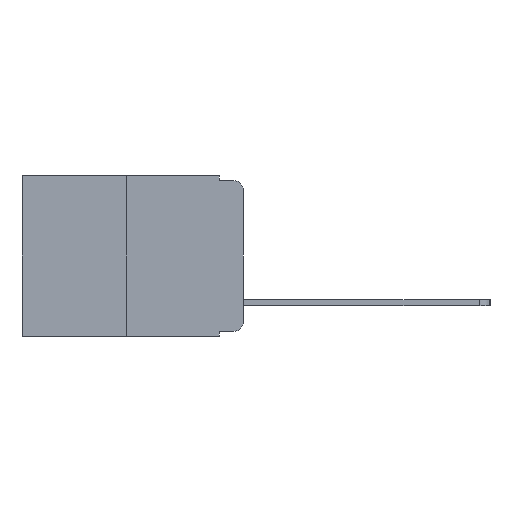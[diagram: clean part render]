
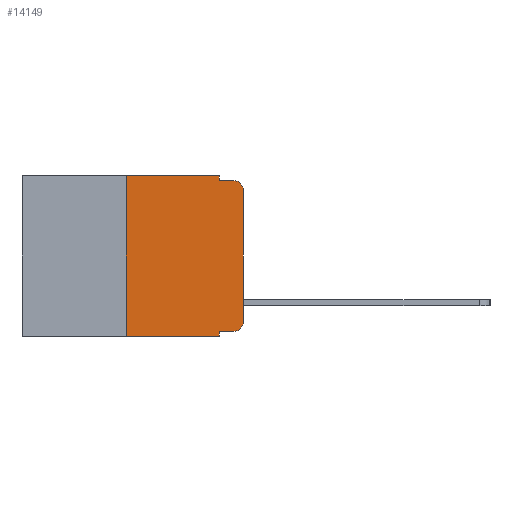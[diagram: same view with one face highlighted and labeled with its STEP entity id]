
A CAD part, left-side view. The second image highlights one B-rep face of the part: STEP entity #14149.
In plain terms, the highlighted planar face has unit normal (-1, 0, 0).
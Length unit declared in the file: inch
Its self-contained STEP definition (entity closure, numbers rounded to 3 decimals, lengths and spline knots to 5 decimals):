
#68 = CARTESIAN_POINT ( 'NONE',  ( 0., 0.473, -0.343 ) ) ;
#138 = DIRECTION ( 'NONE',  ( -1., 0., 0. ) ) ;
#363 = VECTOR ( 'NONE', #20311, 39.37008 ) ;
#501 = EDGE_CURVE ( 'NONE', #15374, #21090, #3777, .T. ) ;
#594 = CARTESIAN_POINT ( 'NONE',  ( 0., 0.02, -0.03 ) ) ;
#913 = ORIENTED_EDGE ( 'NONE', *, *, #1775, .T. ) ;
#965 = DIRECTION ( 'NONE',  ( 0., 0., -1. ) ) ;
#1468 = CIRCLE ( 'NONE', #21874, 0.02 ) ;
#1775 = EDGE_CURVE ( 'NONE', #3227, #13950, #23199, .T. ) ;
#1948 = VECTOR ( 'NONE', #9730, 39.37008 ) ;
#2402 = ORIENTED_EDGE ( 'NONE', *, *, #15412, .T. ) ;
#2527 = DIRECTION ( 'NONE',  ( 0., 0., -1. ) ) ;
#2558 = CARTESIAN_POINT ( 'NONE',  ( 0., 0.02, -0.333 ) ) ;
#3049 = EDGE_CURVE ( 'NONE', #13950, #14395, #9987, .T. ) ;
#3227 = VERTEX_POINT ( 'NONE', #12447 ) ;
#3551 = ORIENTED_EDGE ( 'NONE', *, *, #21712, .F. ) ;
#3776 = CARTESIAN_POINT ( 'NONE',  ( 0., 0.051, 0. ) ) ;
#3777 = LINE ( 'NONE', #68, #12321 ) ;
#3799 = LINE ( 'NONE', #8191, #17587 ) ;
#4627 = VERTEX_POINT ( 'NONE', #3776 ) ;
#5317 = DIRECTION ( 'NONE',  ( 0., 0., 1. ) ) ;
#5547 = EDGE_CURVE ( 'NONE', #3227, #21090, #6926, .T. ) ;
#5904 = CARTESIAN_POINT ( 'NONE',  ( 0., 0.051, -0.01 ) ) ;
#5955 = LINE ( 'NONE', #9815, #363 ) ;
#6106 = CARTESIAN_POINT ( 'NONE',  ( 0., 0.25, -0.343 ) ) ;
#6197 = ORIENTED_EDGE ( 'NONE', *, *, #18888, .T. ) ;
#6452 = CARTESIAN_POINT ( 'NONE',  ( 0., 0.051, -0.343 ) ) ;
#6875 = CARTESIAN_POINT ( 'NONE',  ( 0., 0.051, -0.01 ) ) ;
#6926 = LINE ( 'NONE', #7540, #1948 ) ;
#7183 = CARTESIAN_POINT ( 'NONE',  ( 0., 0., 0. ) ) ;
#7217 = VERTEX_POINT ( 'NONE', #16997 ) ;
#7333 = ORIENTED_EDGE ( 'NONE', *, *, #20123, .F. ) ;
#7540 = CARTESIAN_POINT ( 'NONE',  ( 0., 0.051, 0. ) ) ;
#7579 = VECTOR ( 'NONE', #11420, 39.37008 ) ;
#8191 = CARTESIAN_POINT ( 'NONE',  ( 0., 0.051, 0. ) ) ;
#8509 = ORIENTED_EDGE ( 'NONE', *, *, #13890, .F. ) ;
#8701 = DIRECTION ( 'NONE',  ( 0., -1., 0. ) ) ;
#9199 = VERTEX_POINT ( 'NONE', #5904 ) ;
#9230 = EDGE_CURVE ( 'NONE', #15374, #14036, #17061, .T. ) ;
#9583 = CARTESIAN_POINT ( 'NONE',  ( 0., 0.25, 0. ) ) ;
#9623 = ORIENTED_EDGE ( 'NONE', *, *, #5547, .F. ) ;
#9730 = DIRECTION ( 'NONE',  ( 0., 0., -1. ) ) ;
#9788 = VECTOR ( 'NONE', #13417, 39.37008 ) ;
#9815 = CARTESIAN_POINT ( 'NONE',  ( 0., 0.473, 0. ) ) ;
#9987 = CIRCLE ( 'NONE', #18444, 0.02 ) ;
#10115 = CARTESIAN_POINT ( 'NONE',  ( 0., 0.25, 0. ) ) ;
#10413 = DIRECTION ( 'NONE',  ( 1., 0., 0. ) ) ;
#10709 = ORIENTED_EDGE ( 'NONE', *, *, #3049, .T. ) ;
#11010 = LINE ( 'NONE', #6875, #15202 ) ;
#11275 = LINE ( 'NONE', #7183, #20554 ) ;
#11420 = DIRECTION ( 'NONE',  ( 0., 0., 1. ) ) ;
#12321 = VECTOR ( 'NONE', #15116, 39.37008 ) ;
#12447 = CARTESIAN_POINT ( 'NONE',  ( 0., 0.051, -0.333 ) ) ;
#13417 = DIRECTION ( 'NONE',  ( 0., -1., 0. ) ) ;
#13430 = DIRECTION ( 'NONE',  ( -1., 0., 0. ) ) ;
#13665 = CARTESIAN_POINT ( 'NONE',  ( 0., 0.051, -0.333 ) ) ;
#13784 = ORIENTED_EDGE ( 'NONE', *, *, #9230, .F. ) ;
#13890 = EDGE_CURVE ( 'NONE', #14036, #4627, #5955, .T. ) ;
#13950 = VERTEX_POINT ( 'NONE', #2558 ) ;
#14036 = VERTEX_POINT ( 'NONE', #10115 ) ;
#14149 = ADVANCED_FACE ( 'NONE', ( #15767 ), #19177, .F. ) ;
#14395 = VERTEX_POINT ( 'NONE', #21133 ) ;
#15116 = DIRECTION ( 'NONE',  ( 0., -1., 0. ) ) ;
#15202 = VECTOR ( 'NONE', #8701, 39.37008 ) ;
#15374 = VERTEX_POINT ( 'NONE', #6106 ) ;
#15412 = EDGE_CURVE ( 'NONE', #21756, #7217, #1468, .T. ) ;
#15767 = FACE_OUTER_BOUND ( 'NONE', #20485, .T. ) ;
#16997 = CARTESIAN_POINT ( 'NONE',  ( 0., 0.02, -0.01 ) ) ;
#17061 = LINE ( 'NONE', #9583, #7579 ) ;
#17587 = VECTOR ( 'NONE', #22250, 39.37008 ) ;
#18433 = CARTESIAN_POINT ( 'NONE',  ( 0., 0.02, -0.313 ) ) ;
#18444 = AXIS2_PLACEMENT_3D ( 'NONE', #18433, #138, #965 ) ;
#18888 = EDGE_CURVE ( 'NONE', #14395, #21756, #11275, .T. ) ;
#18913 = CARTESIAN_POINT ( 'NONE',  ( 0., 0., -0.03 ) ) ;
#19177 = PLANE ( 'NONE',  #20121 ) ;
#20121 = AXIS2_PLACEMENT_3D ( 'NONE', #20901, #10413, #22683 ) ;
#20123 = EDGE_CURVE ( 'NONE', #9199, #7217, #11010, .T. ) ;
#20311 = DIRECTION ( 'NONE',  ( 0., -1., 0. ) ) ;
#20485 = EDGE_LOOP ( 'NONE', ( #6197, #2402, #7333, #3551, #8509, #13784, #23047, #9623, #913, #10709 ) ) ;
#20554 = VECTOR ( 'NONE', #5317, 39.37008 ) ;
#20901 = CARTESIAN_POINT ( 'NONE',  ( 0., 0.473, 0. ) ) ;
#21090 = VERTEX_POINT ( 'NONE', #6452 ) ;
#21133 = CARTESIAN_POINT ( 'NONE',  ( 0., 0., -0.313 ) ) ;
#21712 = EDGE_CURVE ( 'NONE', #4627, #9199, #3799, .T. ) ;
#21756 = VERTEX_POINT ( 'NONE', #18913 ) ;
#21874 = AXIS2_PLACEMENT_3D ( 'NONE', #594, #13430, #2527 ) ;
#22250 = DIRECTION ( 'NONE',  ( 0., 0., -1. ) ) ;
#22683 = DIRECTION ( 'NONE',  ( 0., 0., -1. ) ) ;
#23047 = ORIENTED_EDGE ( 'NONE', *, *, #501, .T. ) ;
#23199 = LINE ( 'NONE', #13665, #9788 ) ;
